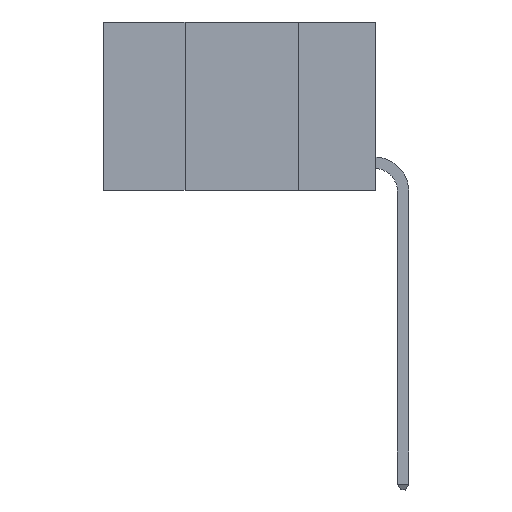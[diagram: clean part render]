
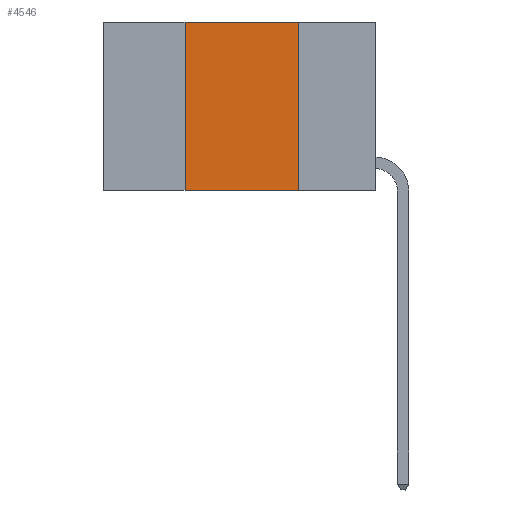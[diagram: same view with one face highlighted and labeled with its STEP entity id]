
A CAD part, left-side view. The second image highlights one B-rep face of the part: STEP entity #4546.
In plain terms, the highlighted planar face has unit normal (-1, 0, 0).
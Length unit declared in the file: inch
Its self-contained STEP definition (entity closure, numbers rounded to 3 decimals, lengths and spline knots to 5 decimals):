
#103 = VECTOR ( 'NONE', #10497, 39.37008 ) ;
#383 = CARTESIAN_POINT ( 'NONE',  ( 0., 0.42, -0.37 ) ) ;
#470 = FACE_OUTER_BOUND ( 'NONE', #1645, .T. ) ;
#1116 = VERTEX_POINT ( 'NONE', #1273 ) ;
#1273 = CARTESIAN_POINT ( 'NONE',  ( 0., 0.42, 0. ) ) ;
#1537 = VECTOR ( 'NONE', #11349, 39.37008 ) ;
#1645 = EDGE_LOOP ( 'NONE', ( #2707, #3788, #5961, #11606 ) ) ;
#2336 = EDGE_CURVE ( 'NONE', #10054, #1116, #2786, .T. ) ;
#2707 = ORIENTED_EDGE ( 'NONE', *, *, #10025, .F. ) ;
#2744 = DIRECTION ( 'NONE',  ( 0., 0., -1. ) ) ;
#2759 = DIRECTION ( 'NONE',  ( 1., 0., 0. ) ) ;
#2783 = PLANE ( 'NONE',  #12249 ) ;
#2786 = LINE ( 'NONE', #10839, #103 ) ;
#2832 = CARTESIAN_POINT ( 'NONE',  ( 0., 0.6, 0. ) ) ;
#3009 = EDGE_CURVE ( 'NONE', #1116, #7311, #9478, .T. ) ;
#3788 = ORIENTED_EDGE ( 'NONE', *, *, #3009, .F. ) ;
#4263 = VECTOR ( 'NONE', #10280, 39.37008 ) ;
#4546 = ADVANCED_FACE ( 'NONE', ( #470 ), #2783, .F. ) ;
#4957 = CARTESIAN_POINT ( 'NONE',  ( 0., 0.17, 0. ) ) ;
#5594 = CARTESIAN_POINT ( 'NONE',  ( 0., 0.6, -0.37 ) ) ;
#5961 = ORIENTED_EDGE ( 'NONE', *, *, #2336, .F. ) ;
#7122 = LINE ( 'NONE', #7493, #4263 ) ;
#7311 = VERTEX_POINT ( 'NONE', #4957 ) ;
#7493 = CARTESIAN_POINT ( 'NONE',  ( 0., 0.17, 0. ) ) ;
#7852 = CARTESIAN_POINT ( 'NONE',  ( 0., 0.17, -0.37 ) ) ;
#8776 = VECTOR ( 'NONE', #12259, 39.37008 ) ;
#9078 = LINE ( 'NONE', #5594, #8776 ) ;
#9478 = LINE ( 'NONE', #11671, #1537 ) ;
#9593 = VERTEX_POINT ( 'NONE', #7852 ) ;
#10025 = EDGE_CURVE ( 'NONE', #7311, #9593, #7122, .T. ) ;
#10054 = VERTEX_POINT ( 'NONE', #383 ) ;
#10280 = DIRECTION ( 'NONE',  ( 0., 0., -1. ) ) ;
#10497 = DIRECTION ( 'NONE',  ( 0., 0., 1. ) ) ;
#10839 = CARTESIAN_POINT ( 'NONE',  ( 0., 0.42, 0. ) ) ;
#11349 = DIRECTION ( 'NONE',  ( 0., -1., 0. ) ) ;
#11606 = ORIENTED_EDGE ( 'NONE', *, *, #12284, .T. ) ;
#11671 = CARTESIAN_POINT ( 'NONE',  ( 0., 0.6, 0. ) ) ;
#12249 = AXIS2_PLACEMENT_3D ( 'NONE', #2832, #2759, #2744 ) ;
#12259 = DIRECTION ( 'NONE',  ( 0., -1., 0. ) ) ;
#12284 = EDGE_CURVE ( 'NONE', #10054, #9593, #9078, .T. ) ;
